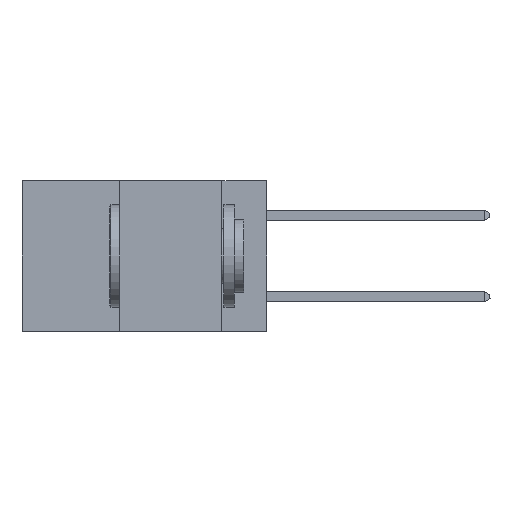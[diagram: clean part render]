
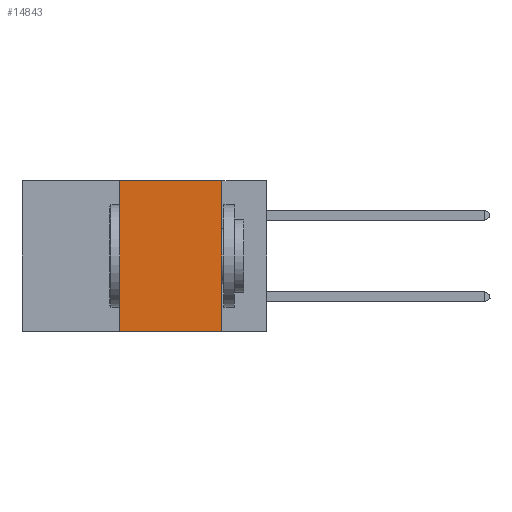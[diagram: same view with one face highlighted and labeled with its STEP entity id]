
A CAD part, left-side view. The second image highlights one B-rep face of the part: STEP entity #14843.
In plain terms, the highlighted planar face has unit normal (-1, 0, 0).
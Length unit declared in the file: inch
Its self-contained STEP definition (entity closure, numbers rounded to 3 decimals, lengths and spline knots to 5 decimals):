
#776 = ORIENTED_EDGE ( 'NONE', *, *, #22284, .T. ) ;
#1009 = LINE ( 'NONE', #5183, #11094 ) ;
#2680 = LINE ( 'NONE', #22350, #15579 ) ;
#2687 = EDGE_LOOP ( 'NONE', ( #22098, #11853, #22425, #776 ) ) ;
#4358 = EDGE_CURVE ( 'NONE', #22330, #16966, #12117, .T. ) ;
#4426 = DIRECTION ( 'NONE',  ( 0., 0., -1. ) ) ;
#4664 = CARTESIAN_POINT ( 'NONE',  ( 0., 0.36, -0.37 ) ) ;
#5183 = CARTESIAN_POINT ( 'NONE',  ( 0., 0.6, -0.37 ) ) ;
#7290 = CARTESIAN_POINT ( 'NONE',  ( 0., 0.36, 0. ) ) ;
#11094 = VECTOR ( 'NONE', #20807, 39.37008 ) ;
#11319 = CARTESIAN_POINT ( 'NONE',  ( 0., 0.11, -0.37 ) ) ;
#11741 = CARTESIAN_POINT ( 'NONE',  ( 0., 0.6, 0. ) ) ;
#11853 = ORIENTED_EDGE ( 'NONE', *, *, #4358, .F. ) ;
#12117 = LINE ( 'NONE', #11741, #23207 ) ;
#13549 = VERTEX_POINT ( 'NONE', #4664 ) ;
#13765 = AXIS2_PLACEMENT_3D ( 'NONE', #21309, #17173, #28263 ) ;
#14086 = DIRECTION ( 'NONE',  ( 0., -1., 0. ) ) ;
#14268 = LINE ( 'NONE', #7290, #15665 ) ;
#14843 = ADVANCED_FACE ( 'NONE', ( #27335 ), #16979, .F. ) ;
#15421 = CARTESIAN_POINT ( 'NONE',  ( 0., 0.11, 0. ) ) ;
#15579 = VECTOR ( 'NONE', #4426, 39.37008 ) ;
#15665 = VECTOR ( 'NONE', #22813, 39.37008 ) ;
#16966 = VERTEX_POINT ( 'NONE', #15421 ) ;
#16979 = PLANE ( 'NONE',  #13765 ) ;
#17173 = DIRECTION ( 'NONE',  ( 1., 0., 0. ) ) ;
#18120 = EDGE_CURVE ( 'NONE', #13549, #22330, #14268, .T. ) ;
#20807 = DIRECTION ( 'NONE',  ( 0., -1., 0. ) ) ;
#21309 = CARTESIAN_POINT ( 'NONE',  ( 0., 0.6, 0. ) ) ;
#22098 = ORIENTED_EDGE ( 'NONE', *, *, #27953, .F. ) ;
#22284 = EDGE_CURVE ( 'NONE', #13549, #27383, #1009, .T. ) ;
#22330 = VERTEX_POINT ( 'NONE', #27465 ) ;
#22350 = CARTESIAN_POINT ( 'NONE',  ( 0., 0.11, 0. ) ) ;
#22425 = ORIENTED_EDGE ( 'NONE', *, *, #18120, .F. ) ;
#22813 = DIRECTION ( 'NONE',  ( 0., 0., 1. ) ) ;
#23207 = VECTOR ( 'NONE', #14086, 39.37008 ) ;
#27335 = FACE_OUTER_BOUND ( 'NONE', #2687, .T. ) ;
#27383 = VERTEX_POINT ( 'NONE', #11319 ) ;
#27465 = CARTESIAN_POINT ( 'NONE',  ( 0., 0.36, 0. ) ) ;
#27953 = EDGE_CURVE ( 'NONE', #16966, #27383, #2680, .T. ) ;
#28263 = DIRECTION ( 'NONE',  ( 0., 0., -1. ) ) ;
